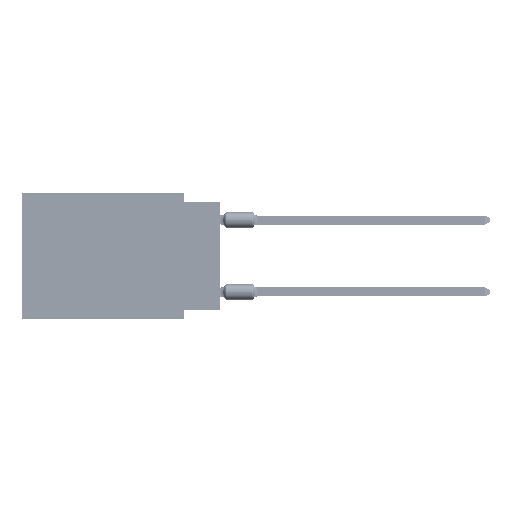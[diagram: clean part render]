
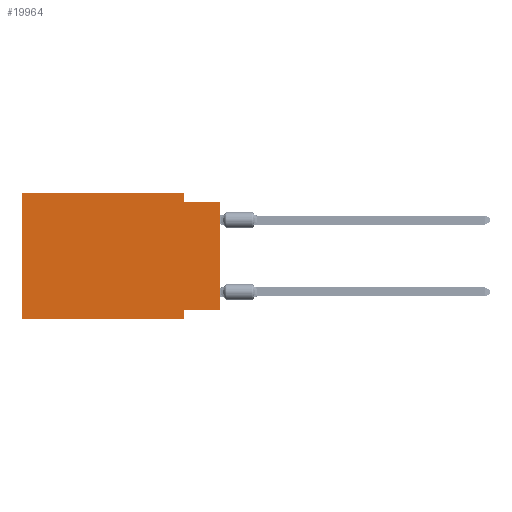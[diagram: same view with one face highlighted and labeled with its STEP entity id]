
A CAD part, left-side view. The second image highlights one B-rep face of the part: STEP entity #19964.
In plain terms, the highlighted planar face has unit normal (-1, 0, 0).
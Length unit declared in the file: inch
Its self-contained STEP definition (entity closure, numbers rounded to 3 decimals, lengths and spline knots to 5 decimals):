
#238 = VECTOR ( 'NONE', #18592, 39.37008 ) ;
#2251 = VECTOR ( 'NONE', #74558, 39.37008 ) ;
#2950 = CARTESIAN_POINT ( 'NONE',  ( 0., 0.55, 0. ) ) ;
#4222 = CARTESIAN_POINT ( 'NONE',  ( 0., 0., -0.325 ) ) ;
#4341 = LINE ( 'NONE', #83633, #238 ) ;
#5274 = DIRECTION ( 'NONE',  ( 0., -1., 0. ) ) ;
#5732 = CARTESIAN_POINT ( 'NONE',  ( 0., 0.1, 0. ) ) ;
#6604 = VERTEX_POINT ( 'NONE', #46450 ) ;
#6872 = CARTESIAN_POINT ( 'NONE',  ( 0., 0.55, 0. ) ) ;
#6971 = ORIENTED_EDGE ( 'NONE', *, *, #84389, .F. ) ;
#7630 = EDGE_CURVE ( 'NONE', #48029, #53610, #4341, .T. ) ;
#10075 = VERTEX_POINT ( 'NONE', #2950 ) ;
#10336 = VERTEX_POINT ( 'NONE', #18613 ) ;
#11394 = LINE ( 'NONE', #71141, #78744 ) ;
#11843 = CARTESIAN_POINT ( 'NONE',  ( 0., 0., -0.025 ) ) ;
#13406 = LINE ( 'NONE', #14243, #46038 ) ;
#13723 = PLANE ( 'NONE',  #40349 ) ;
#14243 = CARTESIAN_POINT ( 'NONE',  ( 0., 0.55, 0. ) ) ;
#14877 = ORIENTED_EDGE ( 'NONE', *, *, #63596, .F. ) ;
#15281 = VECTOR ( 'NONE', #37588, 39.37008 ) ;
#16982 = ORIENTED_EDGE ( 'NONE', *, *, #73368, .F. ) ;
#18592 = DIRECTION ( 'NONE',  ( 0., 1., 0. ) ) ;
#18613 = CARTESIAN_POINT ( 'NONE',  ( 0., 0.1, -0.025 ) ) ;
#18872 = ORIENTED_EDGE ( 'NONE', *, *, #64410, .F. ) ;
#19964 = ADVANCED_FACE ( 'NONE', ( #82696 ), #13723, .F. ) ;
#20262 = DIRECTION ( 'NONE',  ( 1., 0., 0. ) ) ;
#20782 = DIRECTION ( 'NONE',  ( 0., 0., 1. ) ) ;
#23270 = EDGE_LOOP ( 'NONE', ( #47693, #18872, #52117, #16982, #14877, #47372, #6971, #76985 ) ) ;
#25598 = VECTOR ( 'NONE', #5274, 39.37008 ) ;
#32185 = VERTEX_POINT ( 'NONE', #70163 ) ;
#37588 = DIRECTION ( 'NONE',  ( 0., 0., 1. ) ) ;
#39687 = LINE ( 'NONE', #11843, #25598 ) ;
#40349 = AXIS2_PLACEMENT_3D ( 'NONE', #6872, #20262, #65898 ) ;
#41265 = VECTOR ( 'NONE', #77598, 39.37008 ) ;
#41573 = CARTESIAN_POINT ( 'NONE',  ( 0., 0.1, 0. ) ) ;
#42046 = CARTESIAN_POINT ( 'NONE',  ( 0., 0.55, 0. ) ) ;
#45181 = LINE ( 'NONE', #42046, #2251 ) ;
#46038 = VECTOR ( 'NONE', #20782, 39.37008 ) ;
#46450 = CARTESIAN_POINT ( 'NONE',  ( 0., 0., -0.025 ) ) ;
#47372 = ORIENTED_EDGE ( 'NONE', *, *, #65609, .T. ) ;
#47693 = ORIENTED_EDGE ( 'NONE', *, *, #66035, .T. ) ;
#47933 = LINE ( 'NONE', #63849, #15281 ) ;
#48013 = VECTOR ( 'NONE', #59628, 39.37008 ) ;
#48029 = VERTEX_POINT ( 'NONE', #4222 ) ;
#50055 = LINE ( 'NONE', #53091, #48013 ) ;
#52117 = ORIENTED_EDGE ( 'NONE', *, *, #80607, .F. ) ;
#53091 = CARTESIAN_POINT ( 'NONE',  ( 0., 0.55, -0.35 ) ) ;
#53414 = VERTEX_POINT ( 'NONE', #41573 ) ;
#53610 = VERTEX_POINT ( 'NONE', #69236 ) ;
#58628 = LINE ( 'NONE', #5732, #41265 ) ;
#59628 = DIRECTION ( 'NONE',  ( 0., -1., 0. ) ) ;
#63596 = EDGE_CURVE ( 'NONE', #69620, #10075, #13406, .T. ) ;
#63849 = CARTESIAN_POINT ( 'NONE',  ( 0., 0., 0. ) ) ;
#64410 = EDGE_CURVE ( 'NONE', #10336, #6604, #39687, .T. ) ;
#65609 = EDGE_CURVE ( 'NONE', #69620, #32185, #50055, .T. ) ;
#65898 = DIRECTION ( 'NONE',  ( 0., 0., -1. ) ) ;
#66035 = EDGE_CURVE ( 'NONE', #48029, #6604, #47933, .T. ) ;
#66168 = CARTESIAN_POINT ( 'NONE',  ( 0., 0.55, -0.35 ) ) ;
#69236 = CARTESIAN_POINT ( 'NONE',  ( 0., 0.1, -0.325 ) ) ;
#69620 = VERTEX_POINT ( 'NONE', #66168 ) ;
#70163 = CARTESIAN_POINT ( 'NONE',  ( 0., 0.1, -0.35 ) ) ;
#71141 = CARTESIAN_POINT ( 'NONE',  ( 0., 0.1, -0.35 ) ) ;
#73368 = EDGE_CURVE ( 'NONE', #10075, #53414, #45181, .T. ) ;
#74558 = DIRECTION ( 'NONE',  ( 0., -1., 0. ) ) ;
#76985 = ORIENTED_EDGE ( 'NONE', *, *, #7630, .F. ) ;
#77598 = DIRECTION ( 'NONE',  ( 0., 0., -1. ) ) ;
#78744 = VECTOR ( 'NONE', #84229, 39.37008 ) ;
#80607 = EDGE_CURVE ( 'NONE', #53414, #10336, #58628, .T. ) ;
#82696 = FACE_OUTER_BOUND ( 'NONE', #23270, .T. ) ;
#83633 = CARTESIAN_POINT ( 'NONE',  ( 0., 0., -0.325 ) ) ;
#84229 = DIRECTION ( 'NONE',  ( 0., 0., -1. ) ) ;
#84389 = EDGE_CURVE ( 'NONE', #53610, #32185, #11394, .T. ) ;
